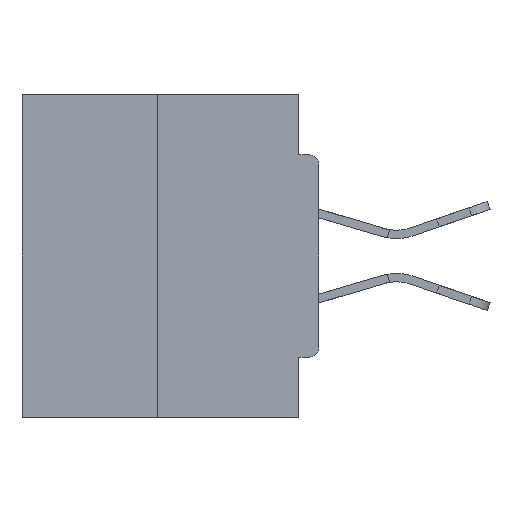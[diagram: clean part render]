
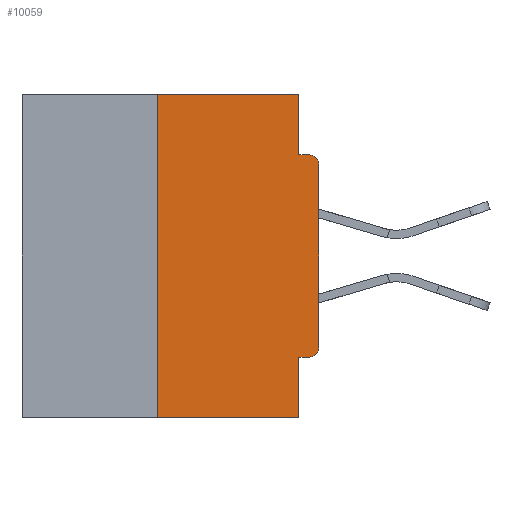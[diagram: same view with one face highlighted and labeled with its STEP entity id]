
A CAD part, left-side view. The second image highlights one B-rep face of the part: STEP entity #10059.
In plain terms, the highlighted planar face has unit normal (-1, 0, 0).
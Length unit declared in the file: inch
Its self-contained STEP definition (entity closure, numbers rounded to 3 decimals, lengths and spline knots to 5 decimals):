
#323 = CARTESIAN_POINT ( 'NONE',  ( 0., 0.25, 0. ) ) ;
#872 = ORIENTED_EDGE ( 'NONE', *, *, #2629, .T. ) ;
#2043 = VERTEX_POINT ( 'NONE', #4927 ) ;
#2629 = EDGE_CURVE ( 'NONE', #33154, #24124, #30828, .T. ) ;
#2816 = EDGE_CURVE ( 'NONE', #11346, #17405, #32245, .T. ) ;
#3131 = DIRECTION ( 'NONE',  ( 0., 1., 0. ) ) ;
#3782 = ORIENTED_EDGE ( 'NONE', *, *, #13993, .F. ) ;
#3994 = VECTOR ( 'NONE', #10859, 39.37008 ) ;
#4325 = VERTEX_POINT ( 'NONE', #33926 ) ;
#4676 = CARTESIAN_POINT ( 'NONE',  ( 0., 0., -0.3915 ) ) ;
#4758 = DIRECTION ( 'NONE',  ( 0., 0., -1. ) ) ;
#4927 = CARTESIAN_POINT ( 'NONE',  ( 0., 0.031, -0.4065 ) ) ;
#5543 = EDGE_CURVE ( 'NONE', #34110, #35370, #35890, .T. ) ;
#6068 = LINE ( 'NONE', #25341, #17358 ) ;
#7568 = DIRECTION ( 'NONE',  ( 0., 0., -1. ) ) ;
#7793 = ORIENTED_EDGE ( 'NONE', *, *, #14723, .T. ) ;
#7992 = ORIENTED_EDGE ( 'NONE', *, *, #11794, .T. ) ;
#9844 = DIRECTION ( 'NONE',  ( 0., 0., -1. ) ) ;
#9993 = CARTESIAN_POINT ( 'NONE',  ( 0., 0., 0. ) ) ;
#10059 = ADVANCED_FACE ( 'NONE', ( #32047 ), #21482, .F. ) ;
#10442 = EDGE_CURVE ( 'NONE', #29470, #4325, #21439, .T. ) ;
#10859 = DIRECTION ( 'NONE',  ( 0., 0., 1. ) ) ;
#10977 = CARTESIAN_POINT ( 'NONE',  ( 0., 0.46, 0. ) ) ;
#11346 = VERTEX_POINT ( 'NONE', #28838 ) ;
#11407 = LINE ( 'NONE', #323, #3994 ) ;
#11794 = EDGE_CURVE ( 'NONE', #4325, #17405, #23808, .T. ) ;
#11865 = CARTESIAN_POINT ( 'NONE',  ( 0., 0.031, 0. ) ) ;
#12259 = ORIENTED_EDGE ( 'NONE', *, *, #15368, .F. ) ;
#12331 = CARTESIAN_POINT ( 'NONE',  ( 0., 0.25, -0.5 ) ) ;
#12886 = AXIS2_PLACEMENT_3D ( 'NONE', #13142, #30024, #35132 ) ;
#13142 = CARTESIAN_POINT ( 'NONE',  ( 0., 0.46, 0. ) ) ;
#13309 = DIRECTION ( 'NONE',  ( -1., 0., 0. ) ) ;
#13993 = EDGE_CURVE ( 'NONE', #2043, #24124, #29919, .T. ) ;
#14723 = EDGE_CURVE ( 'NONE', #24086, #29470, #24543, .T. ) ;
#15036 = VECTOR ( 'NONE', #22077, 39.37008 ) ;
#15260 = ORIENTED_EDGE ( 'NONE', *, *, #2816, .F. ) ;
#15368 = EDGE_CURVE ( 'NONE', #24086, #2043, #22401, .T. ) ;
#15524 = CARTESIAN_POINT ( 'NONE',  ( 0., 0., -0.0935 ) ) ;
#16950 = EDGE_CURVE ( 'NONE', #35370, #11346, #6068, .T. ) ;
#17358 = VECTOR ( 'NONE', #35918, 39.37008 ) ;
#17405 = VERTEX_POINT ( 'NONE', #30849 ) ;
#18366 = CARTESIAN_POINT ( 'NONE',  ( 0., 0.25, 0. ) ) ;
#18812 = DIRECTION ( 'NONE',  ( 0., -1., 0. ) ) ;
#19006 = CARTESIAN_POINT ( 'NONE',  ( 0., 0.031, -0.5 ) ) ;
#19935 = ORIENTED_EDGE ( 'NONE', *, *, #16950, .F. ) ;
#21077 = VECTOR ( 'NONE', #28431, 39.37008 ) ;
#21439 = LINE ( 'NONE', #9993, #25064 ) ;
#21470 = DIRECTION ( 'NONE',  ( -1., 0., 0. ) ) ;
#21482 = PLANE ( 'NONE',  #12886 ) ;
#21678 = VECTOR ( 'NONE', #3131, 39.37008 ) ;
#22077 = DIRECTION ( 'NONE',  ( 0., -1., 0. ) ) ;
#22099 = CARTESIAN_POINT ( 'NONE',  ( 0., 0.031, -0.5 ) ) ;
#22401 = LINE ( 'NONE', #33151, #21678 ) ;
#23808 = CIRCLE ( 'NONE', #34861, 0.015 ) ;
#24016 = CARTESIAN_POINT ( 'NONE',  ( 0., 0.015, -0.1085 ) ) ;
#24086 = VERTEX_POINT ( 'NONE', #32106 ) ;
#24124 = VERTEX_POINT ( 'NONE', #19006 ) ;
#24146 = DIRECTION ( 'NONE',  ( 0., 0., 1. ) ) ;
#24543 = CIRCLE ( 'NONE', #29187, 0.015 ) ;
#25064 = VECTOR ( 'NONE', #24146, 39.37008 ) ;
#25341 = CARTESIAN_POINT ( 'NONE',  ( 0., 0.031, 0. ) ) ;
#26689 = EDGE_LOOP ( 'NONE', ( #32740, #28971, #872, #3782, #12259, #7793, #28601, #7992, #15260, #19935 ) ) ;
#27796 = EDGE_CURVE ( 'NONE', #33154, #34110, #11407, .T. ) ;
#28070 = CARTESIAN_POINT ( 'NONE',  ( 0., 0.46, -0.5 ) ) ;
#28431 = DIRECTION ( 'NONE',  ( 0., -1., 0. ) ) ;
#28601 = ORIENTED_EDGE ( 'NONE', *, *, #10442, .T. ) ;
#28838 = CARTESIAN_POINT ( 'NONE',  ( 0., 0.031, -0.0935 ) ) ;
#28971 = ORIENTED_EDGE ( 'NONE', *, *, #27796, .F. ) ;
#29187 = AXIS2_PLACEMENT_3D ( 'NONE', #30011, #21470, #4758 ) ;
#29470 = VERTEX_POINT ( 'NONE', #4676 ) ;
#29919 = LINE ( 'NONE', #22099, #33820 ) ;
#30011 = CARTESIAN_POINT ( 'NONE',  ( 0., 0.015, -0.3915 ) ) ;
#30024 = DIRECTION ( 'NONE',  ( 1., 0., 0. ) ) ;
#30828 = LINE ( 'NONE', #28070, #21077 ) ;
#30849 = CARTESIAN_POINT ( 'NONE',  ( 0., 0.015, -0.0935 ) ) ;
#32047 = FACE_OUTER_BOUND ( 'NONE', #26689, .T. ) ;
#32106 = CARTESIAN_POINT ( 'NONE',  ( 0., 0.015, -0.4065 ) ) ;
#32245 = LINE ( 'NONE', #15524, #34355 ) ;
#32740 = ORIENTED_EDGE ( 'NONE', *, *, #5543, .F. ) ;
#33151 = CARTESIAN_POINT ( 'NONE',  ( 0., 0., -0.4065 ) ) ;
#33154 = VERTEX_POINT ( 'NONE', #12331 ) ;
#33820 = VECTOR ( 'NONE', #7568, 39.37008 ) ;
#33926 = CARTESIAN_POINT ( 'NONE',  ( 0., 0., -0.1085 ) ) ;
#34110 = VERTEX_POINT ( 'NONE', #18366 ) ;
#34355 = VECTOR ( 'NONE', #18812, 39.37008 ) ;
#34861 = AXIS2_PLACEMENT_3D ( 'NONE', #24016, #13309, #9844 ) ;
#35132 = DIRECTION ( 'NONE',  ( 0., 0., -1. ) ) ;
#35370 = VERTEX_POINT ( 'NONE', #11865 ) ;
#35890 = LINE ( 'NONE', #10977, #15036 ) ;
#35918 = DIRECTION ( 'NONE',  ( 0., 0., -1. ) ) ;
